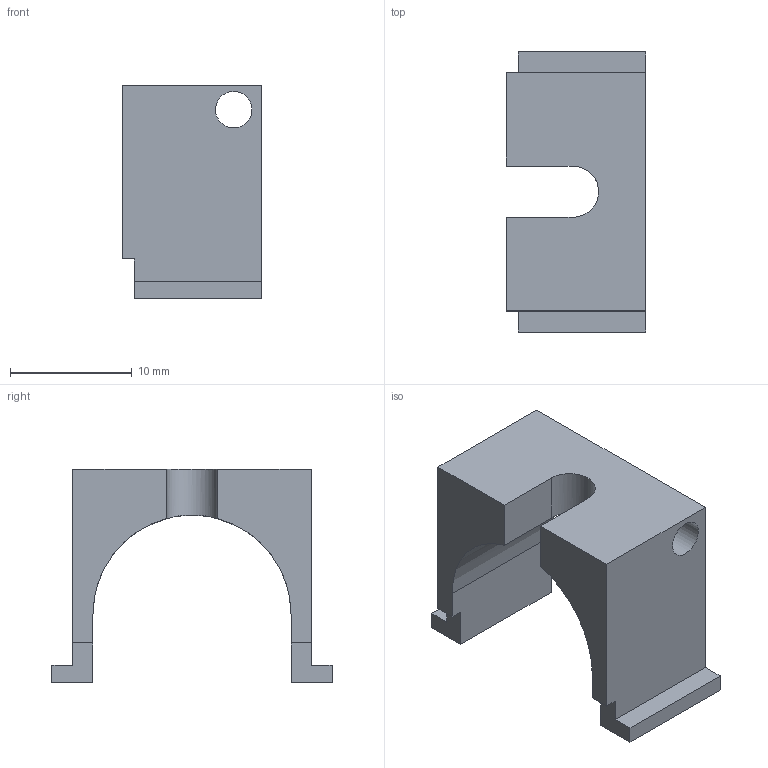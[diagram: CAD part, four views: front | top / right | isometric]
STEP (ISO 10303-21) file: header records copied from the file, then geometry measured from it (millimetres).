
FILE_DESCRIPTION(/* description */ (''),/* implementation_level */ '2;1');
FILE_NAME(/* name */ 'Front Rail Block G26 Updated v2.1.stp',/* time_stamp */ '2021-03-07T00:39:23-06:00',/* author */ ('johne'),/* organization */ (''),/* preprocessor_version */ 'ST-DEVELOPER v18',/* originating_system */ 'Autodesk Inventor 2020',/* authorisation */ '');
FILE_SCHEMA (('AUTOMOTIVE_DESIGN { 1 0 10303 214 3 1 1 }'));
Length unit declared in the file: millimetre
Products named in the file (1): Front Rail Block G26 Updated v2.0
Bounding box: 11.47 x 23 x 17.5 mm (x, y, z)
Volume: 1476.8 mm3; surface area: 1612.8 mm2
Topology: 1 solids, 1 shells, 23 faces, 63 edges, 42 vertices
Faces by surface type: plane 20, cylinder 3
Full cylindrical faces by diameter (mm): 3 x1
Entity records: 814 total; most frequent: CARTESIAN_POINT 146, ORIENTED_EDGE 126, DIRECTION 116, EDGE_CURVE 63, LINE 56, VECTOR 56, VERTEX_POINT 42, AXIS2_PLACEMENT_3D 30
